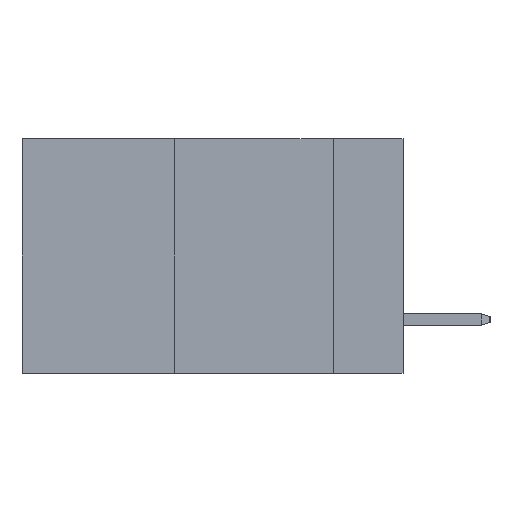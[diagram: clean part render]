
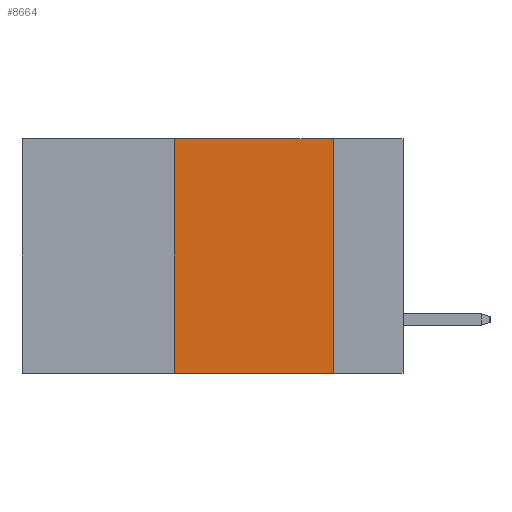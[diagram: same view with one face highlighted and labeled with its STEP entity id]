
A CAD part, left-side view. The second image highlights one B-rep face of the part: STEP entity #8664.
In plain terms, the highlighted planar face has unit normal (-1, 0, 0).
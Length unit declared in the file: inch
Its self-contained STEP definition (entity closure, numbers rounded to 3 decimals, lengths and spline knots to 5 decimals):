
#21 = VERTEX_POINT ( 'NONE', #1195 ) ;
#351 = LINE ( 'NONE', #9388, #5441 ) ;
#375 = DIRECTION ( 'NONE',  ( 0., 0., 1. ) ) ;
#857 = EDGE_CURVE ( 'NONE', #3031, #7166, #5535, .T. ) ;
#1155 = VECTOR ( 'NONE', #9944, 39.37008 ) ;
#1195 = CARTESIAN_POINT ( 'NONE',  ( 0., 0.11, 0. ) ) ;
#1273 = DIRECTION ( 'NONE',  ( 0., -1., 0. ) ) ;
#1461 = CARTESIAN_POINT ( 'NONE',  ( 0., 0.36, 0. ) ) ;
#1547 = ORIENTED_EDGE ( 'NONE', *, *, #4947, .F. ) ;
#1828 = CARTESIAN_POINT ( 'NONE',  ( 0., 0.6, 0. ) ) ;
#2070 = CARTESIAN_POINT ( 'NONE',  ( 0., 0.6, -0.37 ) ) ;
#2931 = LINE ( 'NONE', #5519, #1155 ) ;
#3031 = VERTEX_POINT ( 'NONE', #7269 ) ;
#3391 = DIRECTION ( 'NONE',  ( 1., 0., 0. ) ) ;
#4947 = EDGE_CURVE ( 'NONE', #3031, #6851, #7439, .T. ) ;
#5080 = CARTESIAN_POINT ( 'NONE',  ( 0., 0.11, -0.37 ) ) ;
#5315 = ORIENTED_EDGE ( 'NONE', *, *, #9792, .F. ) ;
#5441 = VECTOR ( 'NONE', #1273, 39.37008 ) ;
#5519 = CARTESIAN_POINT ( 'NONE',  ( 0., 0.11, 0. ) ) ;
#5535 = LINE ( 'NONE', #2070, #9647 ) ;
#6079 = ORIENTED_EDGE ( 'NONE', *, *, #10509, .F. ) ;
#6209 = ORIENTED_EDGE ( 'NONE', *, *, #857, .T. ) ;
#6851 = VERTEX_POINT ( 'NONE', #10662 ) ;
#7117 = AXIS2_PLACEMENT_3D ( 'NONE', #1828, #3391, #10642 ) ;
#7166 = VERTEX_POINT ( 'NONE', #5080 ) ;
#7269 = CARTESIAN_POINT ( 'NONE',  ( 0., 0.36, -0.37 ) ) ;
#7439 = LINE ( 'NONE', #1461, #9189 ) ;
#8287 = EDGE_LOOP ( 'NONE', ( #6079, #5315, #1547, #6209 ) ) ;
#8664 = ADVANCED_FACE ( 'NONE', ( #8836 ), #8669, .F. ) ;
#8669 = PLANE ( 'NONE',  #7117 ) ;
#8836 = FACE_OUTER_BOUND ( 'NONE', #8287, .T. ) ;
#9189 = VECTOR ( 'NONE', #375, 39.37008 ) ;
#9388 = CARTESIAN_POINT ( 'NONE',  ( 0., 0.6, 0. ) ) ;
#9647 = VECTOR ( 'NONE', #10759, 39.37008 ) ;
#9792 = EDGE_CURVE ( 'NONE', #6851, #21, #351, .T. ) ;
#9944 = DIRECTION ( 'NONE',  ( 0., 0., -1. ) ) ;
#10509 = EDGE_CURVE ( 'NONE', #21, #7166, #2931, .T. ) ;
#10642 = DIRECTION ( 'NONE',  ( 0., 0., -1. ) ) ;
#10662 = CARTESIAN_POINT ( 'NONE',  ( 0., 0.36, 0. ) ) ;
#10759 = DIRECTION ( 'NONE',  ( 0., -1., 0. ) ) ;
